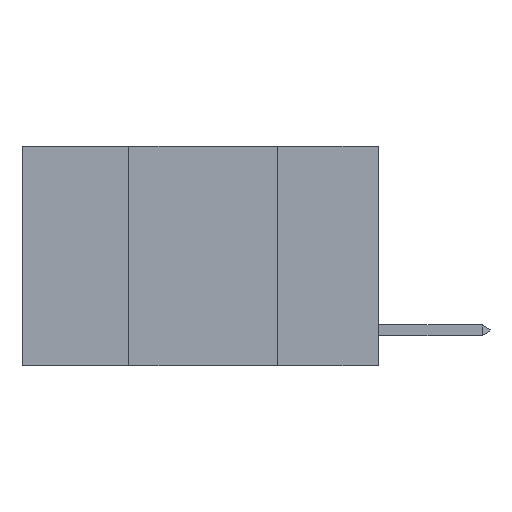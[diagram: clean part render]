
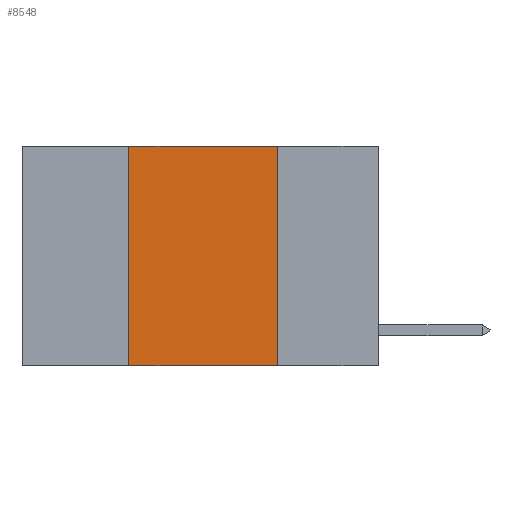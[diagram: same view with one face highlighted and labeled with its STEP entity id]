
A CAD part, left-side view. The second image highlights one B-rep face of the part: STEP entity #8548.
In plain terms, the highlighted planar face has unit normal (-1, 0, 0).
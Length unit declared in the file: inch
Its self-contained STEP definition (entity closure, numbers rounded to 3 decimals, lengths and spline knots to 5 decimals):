
#69 = VERTEX_POINT ( 'NONE', #10184 ) ;
#93 = CARTESIAN_POINT ( 'NONE',  ( 0., 0.17, 0. ) ) ;
#1010 = CARTESIAN_POINT ( 'NONE',  ( 0., 0.6, 0. ) ) ;
#1189 = CARTESIAN_POINT ( 'NONE',  ( 0., 0.6, -0.37 ) ) ;
#1425 = ORIENTED_EDGE ( 'NONE', *, *, #14458, .F. ) ;
#1861 = CARTESIAN_POINT ( 'NONE',  ( 0., 0.17, -0.37 ) ) ;
#2563 = EDGE_CURVE ( 'NONE', #11551, #69, #13335, .T. ) ;
#2695 = CARTESIAN_POINT ( 'NONE',  ( 0., 0.42, 0. ) ) ;
#2956 = VERTEX_POINT ( 'NONE', #93 ) ;
#3296 = DIRECTION ( 'NONE',  ( 0., -1., 0. ) ) ;
#4679 = DIRECTION ( 'NONE',  ( 0., -1., 0. ) ) ;
#4861 = CARTESIAN_POINT ( 'NONE',  ( 0., 0.17, 0. ) ) ;
#5821 = FACE_OUTER_BOUND ( 'NONE', #7775, .T. ) ;
#5932 = LINE ( 'NONE', #1189, #7490 ) ;
#6349 = CARTESIAN_POINT ( 'NONE',  ( 0., 0.42, -0.37 ) ) ;
#6932 = AXIS2_PLACEMENT_3D ( 'NONE', #9412, #15496, #7417 ) ;
#7288 = DIRECTION ( 'NONE',  ( 0., 0., -1. ) ) ;
#7417 = DIRECTION ( 'NONE',  ( 0., 0., -1. ) ) ;
#7490 = VECTOR ( 'NONE', #4679, 39.37008 ) ;
#7775 = EDGE_LOOP ( 'NONE', ( #1425, #15494, #14218, #11658 ) ) ;
#8300 = PLANE ( 'NONE',  #6932 ) ;
#8548 = ADVANCED_FACE ( 'NONE', ( #5821 ), #8300, .F. ) ;
#8589 = LINE ( 'NONE', #4861, #12048 ) ;
#9412 = CARTESIAN_POINT ( 'NONE',  ( 0., 0.6, 0. ) ) ;
#10184 = CARTESIAN_POINT ( 'NONE',  ( 0., 0.42, 0. ) ) ;
#10316 = VECTOR ( 'NONE', #12088, 39.37008 ) ;
#10533 = LINE ( 'NONE', #1010, #11791 ) ;
#11551 = VERTEX_POINT ( 'NONE', #6349 ) ;
#11658 = ORIENTED_EDGE ( 'NONE', *, *, #13539, .T. ) ;
#11791 = VECTOR ( 'NONE', #3296, 39.37008 ) ;
#12048 = VECTOR ( 'NONE', #7288, 39.37008 ) ;
#12088 = DIRECTION ( 'NONE',  ( 0., 0., 1. ) ) ;
#13335 = LINE ( 'NONE', #2695, #10316 ) ;
#13539 = EDGE_CURVE ( 'NONE', #11551, #15477, #5932, .T. ) ;
#13841 = EDGE_CURVE ( 'NONE', #69, #2956, #10533, .T. ) ;
#14218 = ORIENTED_EDGE ( 'NONE', *, *, #2563, .F. ) ;
#14458 = EDGE_CURVE ( 'NONE', #2956, #15477, #8589, .T. ) ;
#15477 = VERTEX_POINT ( 'NONE', #1861 ) ;
#15494 = ORIENTED_EDGE ( 'NONE', *, *, #13841, .F. ) ;
#15496 = DIRECTION ( 'NONE',  ( 1., 0., 0. ) ) ;
